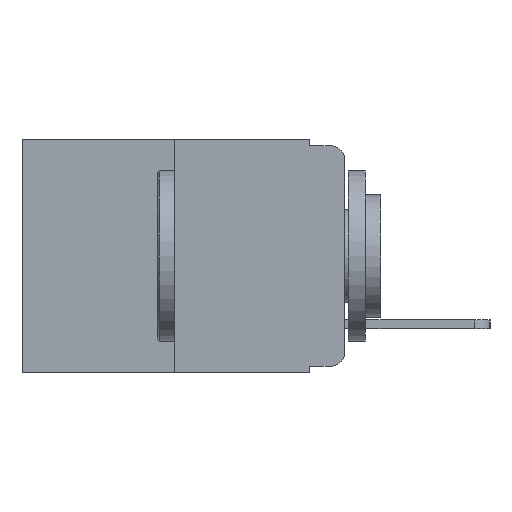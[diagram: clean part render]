
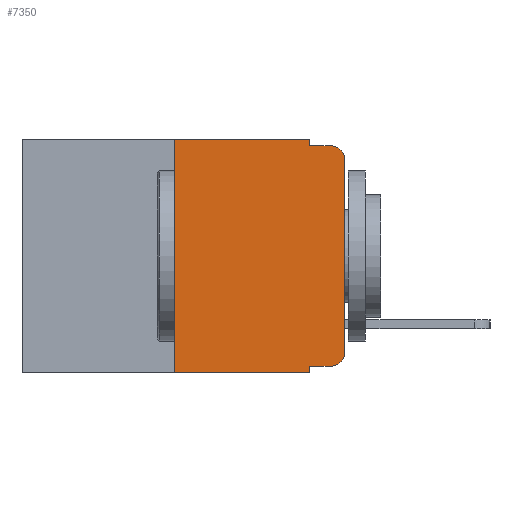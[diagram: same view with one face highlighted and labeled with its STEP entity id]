
A CAD part, left-side view. The second image highlights one B-rep face of the part: STEP entity #7350.
In plain terms, the highlighted planar face has unit normal (-1, 0, 0).
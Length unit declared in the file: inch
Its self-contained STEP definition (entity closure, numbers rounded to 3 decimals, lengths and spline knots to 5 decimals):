
#8 = CARTESIAN_POINT ( 'NONE',  ( 0., 0.25, 0. ) ) ;
#451 = VERTEX_POINT ( 'NONE', #12719 ) ;
#467 = VECTOR ( 'NONE', #1472, 39.37008 ) ;
#691 = DIRECTION ( 'NONE',  ( 0., -1., 0. ) ) ;
#846 = LINE ( 'NONE', #13625, #11908 ) ;
#854 = ORIENTED_EDGE ( 'NONE', *, *, #9542, .T. ) ;
#1388 = LINE ( 'NONE', #12146, #9202 ) ;
#1425 = DIRECTION ( 'NONE',  ( 0., 0., -1. ) ) ;
#1472 = DIRECTION ( 'NONE',  ( 0., 0., 1. ) ) ;
#2270 = AXIS2_PLACEMENT_3D ( 'NONE', #14116, #8148, #1425 ) ;
#2506 = ORIENTED_EDGE ( 'NONE', *, *, #9539, .T. ) ;
#2684 = CARTESIAN_POINT ( 'NONE',  ( 0., 0.051, -0.01 ) ) ;
#2738 = CARTESIAN_POINT ( 'NONE',  ( 0., 0.051, 0. ) ) ;
#2754 = LINE ( 'NONE', #10455, #8862 ) ;
#3041 = CARTESIAN_POINT ( 'NONE',  ( 0., 0.02, -0.313 ) ) ;
#3054 = ORIENTED_EDGE ( 'NONE', *, *, #9494, .F. ) ;
#3131 = VECTOR ( 'NONE', #6174, 39.37008 ) ;
#3288 = CARTESIAN_POINT ( 'NONE',  ( 0., 0.473, 0. ) ) ;
#3734 = VERTEX_POINT ( 'NONE', #11546 ) ;
#3823 = AXIS2_PLACEMENT_3D ( 'NONE', #3041, #10499, #4273 ) ;
#3857 = VECTOR ( 'NONE', #3865, 39.37008 ) ;
#3865 = DIRECTION ( 'NONE',  ( 0., -1., 0. ) ) ;
#3993 = VECTOR ( 'NONE', #4506, 39.37008 ) ;
#4272 = LINE ( 'NONE', #2684, #3857 ) ;
#4273 = DIRECTION ( 'NONE',  ( 0., 0., -1. ) ) ;
#4506 = DIRECTION ( 'NONE',  ( 0., -1., 0. ) ) ;
#5213 = ORIENTED_EDGE ( 'NONE', *, *, #9516, .F. ) ;
#5357 = VECTOR ( 'NONE', #11085, 39.37008 ) ;
#5585 = ORIENTED_EDGE ( 'NONE', *, *, #9477, .F. ) ;
#5593 = VERTEX_POINT ( 'NONE', #13776 ) ;
#5627 = VERTEX_POINT ( 'NONE', #6813 ) ;
#6054 = DIRECTION ( 'NONE',  ( 0., 0., -1. ) ) ;
#6174 = DIRECTION ( 'NONE',  ( 0., 0., -1. ) ) ;
#6208 = EDGE_LOOP ( 'NONE', ( #13177, #7040, #5585, #3054, #9090, #7316, #12151, #5213, #2506, #854 ) ) ;
#6231 = VERTEX_POINT ( 'NONE', #13414 ) ;
#6813 = CARTESIAN_POINT ( 'NONE',  ( 0., 0.051, 0. ) ) ;
#6843 = VERTEX_POINT ( 'NONE', #7865 ) ;
#7017 = CARTESIAN_POINT ( 'NONE',  ( 0., 0., 0. ) ) ;
#7040 = ORIENTED_EDGE ( 'NONE', *, *, #9471, .T. ) ;
#7111 = CIRCLE ( 'NONE', #2270, 0.02 ) ;
#7158 = DIRECTION ( 'NONE',  ( 0., 0., -1. ) ) ;
#7316 = ORIENTED_EDGE ( 'NONE', *, *, #9497, .F. ) ;
#7350 = ADVANCED_FACE ( 'NONE', ( #7417 ), #10119, .F. ) ;
#7355 = VERTEX_POINT ( 'NONE', #13065 ) ;
#7417 = FACE_OUTER_BOUND ( 'NONE', #6208, .T. ) ;
#7492 = VERTEX_POINT ( 'NONE', #8272 ) ;
#7785 = LINE ( 'NONE', #7017, #5357 ) ;
#7865 = CARTESIAN_POINT ( 'NONE',  ( 0., 0.02, -0.333 ) ) ;
#8148 = DIRECTION ( 'NONE',  ( -1., 0., 0. ) ) ;
#8272 = CARTESIAN_POINT ( 'NONE',  ( 0., 0.051, -0.343 ) ) ;
#8532 = CARTESIAN_POINT ( 'NONE',  ( 0., 0.25, -0.343 ) ) ;
#8705 = EDGE_CURVE ( 'NONE', #451, #5627, #9948, .T. ) ;
#8862 = VECTOR ( 'NONE', #9275, 39.37008 ) ;
#8989 = AXIS2_PLACEMENT_3D ( 'NONE', #11091, #12052, #6054 ) ;
#9090 = ORIENTED_EDGE ( 'NONE', *, *, #8705, .F. ) ;
#9202 = VECTOR ( 'NONE', #7158, 39.37008 ) ;
#9234 = EDGE_CURVE ( 'NONE', #9634, #7492, #846, .T. ) ;
#9275 = DIRECTION ( 'NONE',  ( 0., -1., 0. ) ) ;
#9454 = EDGE_CURVE ( 'NONE', #5593, #9770, #7785, .T. ) ;
#9471 = EDGE_CURVE ( 'NONE', #9770, #3734, #7111, .T. ) ;
#9477 = EDGE_CURVE ( 'NONE', #7355, #3734, #4272, .T. ) ;
#9494 = EDGE_CURVE ( 'NONE', #5627, #7355, #1388, .T. ) ;
#9497 = EDGE_CURVE ( 'NONE', #9634, #451, #11803, .T. ) ;
#9516 = EDGE_CURVE ( 'NONE', #6231, #7492, #11515, .T. ) ;
#9539 = EDGE_CURVE ( 'NONE', #6231, #6843, #2754, .T. ) ;
#9542 = EDGE_CURVE ( 'NONE', #6843, #5593, #10908, .T. ) ;
#9634 = VERTEX_POINT ( 'NONE', #8532 ) ;
#9770 = VERTEX_POINT ( 'NONE', #12675 ) ;
#9948 = LINE ( 'NONE', #3288, #3993 ) ;
#10119 = PLANE ( 'NONE',  #8989 ) ;
#10455 = CARTESIAN_POINT ( 'NONE',  ( 0., 0.051, -0.333 ) ) ;
#10499 = DIRECTION ( 'NONE',  ( -1., 0., 0. ) ) ;
#10908 = CIRCLE ( 'NONE', #3823, 0.02 ) ;
#11085 = DIRECTION ( 'NONE',  ( 0., 0., 1. ) ) ;
#11091 = CARTESIAN_POINT ( 'NONE',  ( 0., 0.473, 0. ) ) ;
#11515 = LINE ( 'NONE', #2738, #3131 ) ;
#11546 = CARTESIAN_POINT ( 'NONE',  ( 0., 0.02, -0.01 ) ) ;
#11803 = LINE ( 'NONE', #8, #467 ) ;
#11908 = VECTOR ( 'NONE', #691, 39.37008 ) ;
#12052 = DIRECTION ( 'NONE',  ( 1., 0., 0. ) ) ;
#12146 = CARTESIAN_POINT ( 'NONE',  ( 0., 0.051, 0. ) ) ;
#12151 = ORIENTED_EDGE ( 'NONE', *, *, #9234, .T. ) ;
#12675 = CARTESIAN_POINT ( 'NONE',  ( 0., 0., -0.03 ) ) ;
#12719 = CARTESIAN_POINT ( 'NONE',  ( 0., 0.25, 0. ) ) ;
#13065 = CARTESIAN_POINT ( 'NONE',  ( 0., 0.051, -0.01 ) ) ;
#13177 = ORIENTED_EDGE ( 'NONE', *, *, #9454, .T. ) ;
#13414 = CARTESIAN_POINT ( 'NONE',  ( 0., 0.051, -0.333 ) ) ;
#13625 = CARTESIAN_POINT ( 'NONE',  ( 0., 0.473, -0.343 ) ) ;
#13776 = CARTESIAN_POINT ( 'NONE',  ( 0., 0., -0.313 ) ) ;
#14116 = CARTESIAN_POINT ( 'NONE',  ( 0., 0.02, -0.03 ) ) ;
